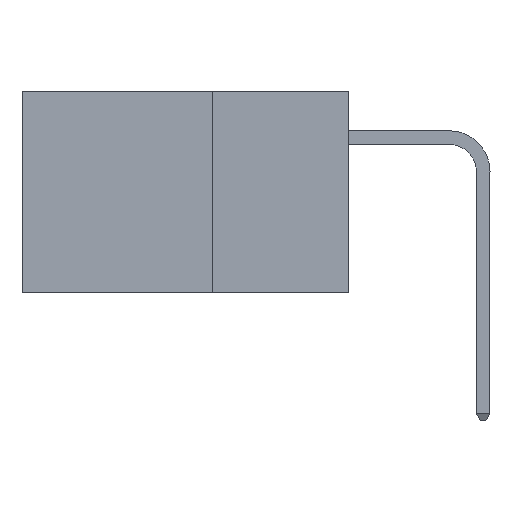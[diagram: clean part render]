
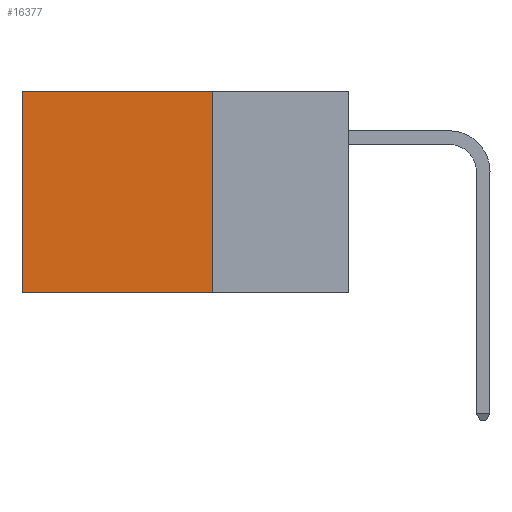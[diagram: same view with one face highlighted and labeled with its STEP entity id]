
A CAD part, left-side view. The second image highlights one B-rep face of the part: STEP entity #16377.
In plain terms, the highlighted planar face has unit normal (-1, 0, 0).
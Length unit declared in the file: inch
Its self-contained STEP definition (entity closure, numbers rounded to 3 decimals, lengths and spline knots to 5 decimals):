
#1071 = CARTESIAN_POINT ( 'NONE',  ( 0.2875, 0.25, 0. ) ) ;
#1215 = AXIS2_PLACEMENT_3D ( 'NONE', #1071, #5078, #14523 ) ;
#1385 = ORIENTED_EDGE ( 'NONE', *, *, #2371, .F. ) ;
#1423 = EDGE_CURVE ( 'NONE', #2297, #5309, #9921, .T. ) ;
#2297 = VERTEX_POINT ( 'NONE', #8272 ) ;
#2332 = CARTESIAN_POINT ( 'NONE',  ( 0.2875, 0.25, -0.37 ) ) ;
#2371 = EDGE_CURVE ( 'NONE', #4302, #4031, #13755, .T. ) ;
#3355 = EDGE_CURVE ( 'NONE', #4031, #5309, #9650, .T. ) ;
#3413 = LINE ( 'NONE', #13636, #6139 ) ;
#4031 = VERTEX_POINT ( 'NONE', #16875 ) ;
#4302 = VERTEX_POINT ( 'NONE', #14183 ) ;
#5078 = DIRECTION ( 'NONE',  ( 1., 0., 0. ) ) ;
#5309 = VERTEX_POINT ( 'NONE', #17015 ) ;
#5367 = ORIENTED_EDGE ( 'NONE', *, *, #7679, .T. ) ;
#5928 = CARTESIAN_POINT ( 'NONE',  ( 0.2875, 0.25, 0. ) ) ;
#6039 = ORIENTED_EDGE ( 'NONE', *, *, #3355, .F. ) ;
#6139 = VECTOR ( 'NONE', #15040, 39.37008 ) ;
#7149 = DIRECTION ( 'NONE',  ( 0., 0., -1. ) ) ;
#7551 = VECTOR ( 'NONE', #11976, 39.37008 ) ;
#7679 = EDGE_CURVE ( 'NONE', #4302, #2297, #3413, .T. ) ;
#8272 = CARTESIAN_POINT ( 'NONE',  ( 0.2875, 0.6, 0. ) ) ;
#9650 = LINE ( 'NONE', #2332, #7551 ) ;
#9921 = LINE ( 'NONE', #16111, #13321 ) ;
#10603 = PLANE ( 'NONE',  #1215 ) ;
#11976 = DIRECTION ( 'NONE',  ( 0., 1., 0. ) ) ;
#11977 = ORIENTED_EDGE ( 'NONE', *, *, #1423, .T. ) ;
#12225 = DIRECTION ( 'NONE',  ( 0., 0., -1. ) ) ;
#13321 = VECTOR ( 'NONE', #12225, 39.37008 ) ;
#13636 = CARTESIAN_POINT ( 'NONE',  ( 0.2875, 0.25, 0. ) ) ;
#13755 = LINE ( 'NONE', #5928, #15427 ) ;
#14183 = CARTESIAN_POINT ( 'NONE',  ( 0.2875, 0.25, 0. ) ) ;
#14294 = EDGE_LOOP ( 'NONE', ( #11977, #6039, #1385, #5367 ) ) ;
#14523 = DIRECTION ( 'NONE',  ( 0., 0., -1. ) ) ;
#15040 = DIRECTION ( 'NONE',  ( 0., 1., 0. ) ) ;
#15238 = FACE_OUTER_BOUND ( 'NONE', #14294, .T. ) ;
#15427 = VECTOR ( 'NONE', #7149, 39.37008 ) ;
#16111 = CARTESIAN_POINT ( 'NONE',  ( 0.2875, 0.6, 0. ) ) ;
#16377 = ADVANCED_FACE ( 'NONE', ( #15238 ), #10603, .F. ) ;
#16875 = CARTESIAN_POINT ( 'NONE',  ( 0.2875, 0.25, -0.37 ) ) ;
#17015 = CARTESIAN_POINT ( 'NONE',  ( 0.2875, 0.6, -0.37 ) ) ;
